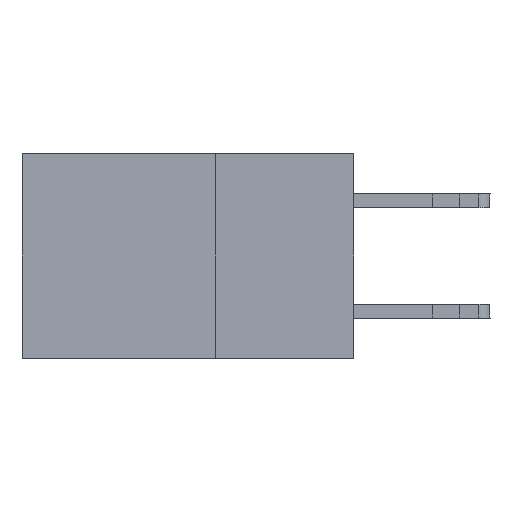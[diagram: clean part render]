
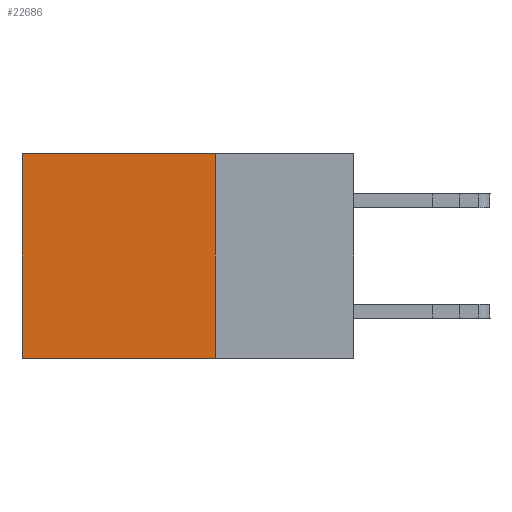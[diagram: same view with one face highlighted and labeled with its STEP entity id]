
A CAD part, left-side view. The second image highlights one B-rep face of the part: STEP entity #22686.
In plain terms, the highlighted planar face has unit normal (-1, 0, 0).
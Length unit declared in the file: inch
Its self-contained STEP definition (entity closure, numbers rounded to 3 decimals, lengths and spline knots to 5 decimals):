
#47 = CARTESIAN_POINT ( 'NONE',  ( 0.2875, 0.6, 0. ) ) ;
#1208 = VERTEX_POINT ( 'NONE', #47 ) ;
#2530 = CARTESIAN_POINT ( 'NONE',  ( 0.2875, 0.25, 0. ) ) ;
#3846 = LINE ( 'NONE', #14562, #16307 ) ;
#7164 = AXIS2_PLACEMENT_3D ( 'NONE', #2530, #28707, #9974 ) ;
#9262 = VECTOR ( 'NONE', #16701, 39.37008 ) ;
#9497 = CARTESIAN_POINT ( 'NONE',  ( 0.2875, 0.25, -0.37 ) ) ;
#9718 = ORIENTED_EDGE ( 'NONE', *, *, #15503, .F. ) ;
#9761 = DIRECTION ( 'NONE',  ( 0., 1., 0. ) ) ;
#9974 = DIRECTION ( 'NONE',  ( 0., 0., -1. ) ) ;
#10748 = ORIENTED_EDGE ( 'NONE', *, *, #15495, .T. ) ;
#10991 = EDGE_LOOP ( 'NONE', ( #24222, #18668, #9718, #10748 ) ) ;
#11252 = FACE_OUTER_BOUND ( 'NONE', #10991, .T. ) ;
#12238 = CARTESIAN_POINT ( 'NONE',  ( 0.2875, 0.6, 0. ) ) ;
#12310 = DIRECTION ( 'NONE',  ( 0., 0., -1. ) ) ;
#14139 = CARTESIAN_POINT ( 'NONE',  ( 0.2875, 0.25, -0.37 ) ) ;
#14562 = CARTESIAN_POINT ( 'NONE',  ( 0.2875, 0.25, 0. ) ) ;
#15495 = EDGE_CURVE ( 'NONE', #27045, #1208, #3846, .T. ) ;
#15503 = EDGE_CURVE ( 'NONE', #27045, #21287, #27997, .T. ) ;
#16307 = VECTOR ( 'NONE', #16965, 39.37008 ) ;
#16360 = PLANE ( 'NONE',  #7164 ) ;
#16701 = DIRECTION ( 'NONE',  ( 0., 0., -1. ) ) ;
#16965 = DIRECTION ( 'NONE',  ( 0., 1., 0. ) ) ;
#18668 = ORIENTED_EDGE ( 'NONE', *, *, #27945, .F. ) ;
#19303 = CARTESIAN_POINT ( 'NONE',  ( 0.2875, 0.25, 0. ) ) ;
#20948 = LINE ( 'NONE', #12238, #9262 ) ;
#21287 = VERTEX_POINT ( 'NONE', #9497 ) ;
#22686 = ADVANCED_FACE ( 'NONE', ( #11252 ), #16360, .F. ) ;
#23798 = VECTOR ( 'NONE', #9761, 39.37008 ) ;
#24222 = ORIENTED_EDGE ( 'NONE', *, *, #26160, .T. ) ;
#25755 = VERTEX_POINT ( 'NONE', #29590 ) ;
#26160 = EDGE_CURVE ( 'NONE', #1208, #25755, #20948, .T. ) ;
#27045 = VERTEX_POINT ( 'NONE', #30282 ) ;
#27945 = EDGE_CURVE ( 'NONE', #21287, #25755, #29686, .T. ) ;
#27997 = LINE ( 'NONE', #19303, #30202 ) ;
#28707 = DIRECTION ( 'NONE',  ( 1., 0., 0. ) ) ;
#29590 = CARTESIAN_POINT ( 'NONE',  ( 0.2875, 0.6, -0.37 ) ) ;
#29686 = LINE ( 'NONE', #14139, #23798 ) ;
#30202 = VECTOR ( 'NONE', #12310, 39.37008 ) ;
#30282 = CARTESIAN_POINT ( 'NONE',  ( 0.2875, 0.25, 0. ) ) ;
